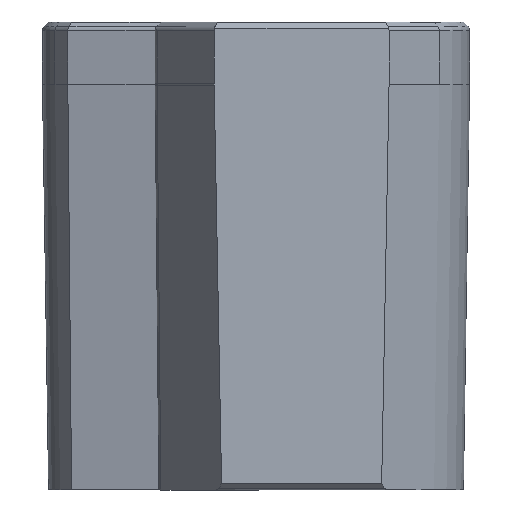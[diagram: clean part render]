
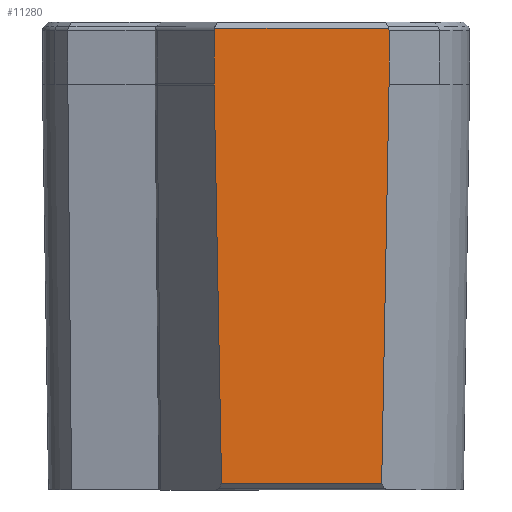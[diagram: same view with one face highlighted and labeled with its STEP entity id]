
A CAD part, left-side view. The second image highlights one B-rep face of the part: STEP entity #11280.
In plain terms, the highlighted planar face has unit normal (-1, 0, 0).
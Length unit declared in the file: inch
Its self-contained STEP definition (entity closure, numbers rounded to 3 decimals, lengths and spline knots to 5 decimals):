
#198 = CARTESIAN_POINT ( 'NONE',  ( -0.683, 0.35555, 2.003 ) ) ;
#259 = VECTOR ( 'NONE', #10219, 39.37008 ) ;
#330 = VECTOR ( 'NONE', #4020, 39.37008 ) ;
#607 = CARTESIAN_POINT ( 'NONE',  ( -0.683, -0.35555, 1.96764 ) ) ;
#680 = EDGE_CURVE ( 'NONE', #5226, #2300, #3069, .T. ) ;
#1098 = CARTESIAN_POINT ( 'NONE',  ( -0.683, -0.34029, 0.925 ) ) ;
#1530 = VERTEX_POINT ( 'NONE', #1868 ) ;
#1868 = CARTESIAN_POINT ( 'NONE',  ( -0.683, 0.35555, 1.96764 ) ) ;
#1951 = VERTEX_POINT ( 'NONE', #11167 ) ;
#2091 = DIRECTION ( 'NONE',  ( 0., 1., 0. ) ) ;
#2143 = CARTESIAN_POINT ( 'NONE',  ( -0.683, 0.35281, 1.978 ) ) ;
#2300 = VERTEX_POINT ( 'NONE', #8418 ) ;
#2865 = CARTESIAN_POINT ( 'NONE',  ( -0.683, 0.35555, 1.978 ) ) ;
#2933 = DIRECTION ( 'NONE',  ( 0., 0., -1. ) ) ;
#2955 = VERTEX_POINT ( 'NONE', #3021 ) ;
#3021 = CARTESIAN_POINT ( 'NONE',  ( -0.683, -0.35555, 1.75 ) ) ;
#3036 = AXIS2_PLACEMENT_3D ( 'NONE', #7751, #3090, #9594 ) ;
#3050 = CARTESIAN_POINT ( 'NONE',  ( -0.683, 0.32549, 0.125 ) ) ;
#3069 = LINE ( 'NONE', #5818, #330 ) ;
#3090 = DIRECTION ( 'NONE',  ( -1., 0., 0. ) ) ;
#3144 = ORIENTED_EDGE ( 'NONE', *, *, #8062, .T. ) ;
#3213 =( BOUNDED_CURVE ( )  B_SPLINE_CURVE ( 3, ( #2143, #5786, #9425, #3990 ),
 .UNSPECIFIED., .F., .T. ) 
 B_SPLINE_CURVE_WITH_KNOTS ( ( 4, 4 ),
 ( 5.85611, 6.28319 ),
 .UNSPECIFIED. ) 
 CURVE ( )  GEOMETRIC_REPRESENTATION_ITEM ( )  RATIONAL_B_SPLINE_CURVE ( ( 1., 0.985, 0.985, 1. ) ) 
 REPRESENTATION_ITEM ( '' )  );
#3379 = VERTEX_POINT ( 'NONE', #7163 ) ;
#3594 = ORIENTED_EDGE ( 'NONE', *, *, #4364, .T. ) ;
#3728 =( BOUNDED_CURVE ( )  B_SPLINE_CURVE ( 3, ( #4738, #5692, #10046, #10289 ),
 .UNSPECIFIED., .F., .T. ) 
 B_SPLINE_CURVE_WITH_KNOTS ( ( 4, 4 ),
 ( 0., 0.01515 ),
 .UNSPECIFIED. ) 
 CURVE ( )  GEOMETRIC_REPRESENTATION_ITEM ( )  RATIONAL_B_SPLINE_CURVE ( ( 1., 1., 1., 1. ) ) 
 REPRESENTATION_ITEM ( '' )  );
#3874 = ORIENTED_EDGE ( 'NONE', *, *, #5268, .F. ) ;
#3990 = CARTESIAN_POINT ( 'NONE',  ( -0.683, 0.35555, 1.96764 ) ) ;
#4020 = DIRECTION ( 'NONE',  ( 0., -1., 0. ) ) ;
#4364 = EDGE_CURVE ( 'NONE', #1951, #1530, #3213, .T. ) ;
#4727 = LINE ( 'NONE', #198, #259 ) ;
#4738 = CARTESIAN_POINT ( 'NONE',  ( -0.683, 0.35555, 1.75379 ) ) ;
#4821 = VECTOR ( 'NONE', #2933, 39.37008 ) ;
#4966 = CARTESIAN_POINT ( 'NONE',  ( -0.683, -0.35555, 1.97123 ) ) ;
#5221 = ORIENTED_EDGE ( 'NONE', *, *, #11648, .F. ) ;
#5226 = VERTEX_POINT ( 'NONE', #3050 ) ;
#5253 = EDGE_CURVE ( 'NONE', #10054, #5226, #8552, .T. ) ;
#5268 = EDGE_CURVE ( 'NONE', #8933, #2955, #8439, .T. ) ;
#5692 = CARTESIAN_POINT ( 'NONE',  ( -0.683, 0.35555, 1.75126 ) ) ;
#5786 = CARTESIAN_POINT ( 'NONE',  ( -0.683, 0.35462, 1.97474 ) ) ;
#5818 = CARTESIAN_POINT ( 'NONE',  ( -0.683, -0.32503, 0.125 ) ) ;
#6097 = CARTESIAN_POINT ( 'NONE',  ( -0.683, -0.35462, 1.97474 ) ) ;
#6282 = LINE ( 'NONE', #1098, #7989 ) ;
#6411 = CARTESIAN_POINT ( 'NONE',  ( -0.683, 0.35555, 1.75379 ) ) ;
#6544 = EDGE_CURVE ( 'NONE', #3379, #1951, #11042, .T. ) ;
#6707 = CARTESIAN_POINT ( 'NONE',  ( -0.683, -0.35555, 2.003 ) ) ;
#7111 = VECTOR ( 'NONE', #10340, 39.37008 ) ;
#7163 = CARTESIAN_POINT ( 'NONE',  ( -0.683, -0.35281, 1.978 ) ) ;
#7381 = ORIENTED_EDGE ( 'NONE', *, *, #5253, .T. ) ;
#7686 = ORIENTED_EDGE ( 'NONE', *, *, #7772, .T. ) ;
#7751 = CARTESIAN_POINT ( 'NONE',  ( -0.683, -0.35555, 1.75 ) ) ;
#7759 = VERTEX_POINT ( 'NONE', #6411 ) ;
#7772 = EDGE_CURVE ( 'NONE', #7759, #10054, #3728, .T. ) ;
#7970 = ORIENTED_EDGE ( 'NONE', *, *, #9845, .T. ) ;
#7989 = VECTOR ( 'NONE', #9917, 39.37008 ) ;
#8062 = EDGE_CURVE ( 'NONE', #8933, #3379, #11055, .T. ) ;
#8418 = CARTESIAN_POINT ( 'NONE',  ( -0.683, -0.32549, 0.125 ) ) ;
#8439 = LINE ( 'NONE', #6707, #4821 ) ;
#8530 = FACE_OUTER_BOUND ( 'NONE', #9222, .T. ) ;
#8552 = LINE ( 'NONE', #9382, #7111 ) ;
#8933 = VERTEX_POINT ( 'NONE', #10229 ) ;
#9096 = ORIENTED_EDGE ( 'NONE', *, *, #680, .T. ) ;
#9222 = EDGE_LOOP ( 'NONE', ( #7970, #7686, #7381, #9096, #5221, #3874, #3144, #9751, #3594 ) ) ;
#9382 = CARTESIAN_POINT ( 'NONE',  ( -0.683, 0.34029, 0.925 ) ) ;
#9425 = CARTESIAN_POINT ( 'NONE',  ( -0.683, 0.35555, 1.97123 ) ) ;
#9555 = VECTOR ( 'NONE', #2091, 39.37008 ) ;
#9594 = DIRECTION ( 'NONE',  ( 0., 1., 0. ) ) ;
#9751 = ORIENTED_EDGE ( 'NONE', *, *, #6544, .T. ) ;
#9845 = EDGE_CURVE ( 'NONE', #1530, #7759, #4727, .T. ) ;
#9917 = DIRECTION ( 'NONE',  ( 0., 0.018, -1. ) ) ;
#10046 = CARTESIAN_POINT ( 'NONE',  ( -0.683, 0.35552, 1.74874 ) ) ;
#10054 = VERTEX_POINT ( 'NONE', #10845 ) ;
#10219 = DIRECTION ( 'NONE',  ( 0., 0., -1. ) ) ;
#10229 = CARTESIAN_POINT ( 'NONE',  ( -0.683, -0.35555, 1.96764 ) ) ;
#10289 = CARTESIAN_POINT ( 'NONE',  ( -0.683, 0.35548, 1.74621 ) ) ;
#10340 = DIRECTION ( 'NONE',  ( 0., -0.018, -1. ) ) ;
#10405 = CARTESIAN_POINT ( 'NONE',  ( -0.683, -0.35281, 1.978 ) ) ;
#10845 = CARTESIAN_POINT ( 'NONE',  ( -0.683, 0.35548, 1.74621 ) ) ;
#11042 = LINE ( 'NONE', #2865, #9555 ) ;
#11055 =( BOUNDED_CURVE ( )  B_SPLINE_CURVE ( 3, ( #607, #4966, #6097, #10405 ),
 .UNSPECIFIED., .F., .T. ) 
 B_SPLINE_CURVE_WITH_KNOTS ( ( 4, 4 ),
 ( 3.14159, 3.56867 ),
 .UNSPECIFIED. ) 
 CURVE ( )  GEOMETRIC_REPRESENTATION_ITEM ( )  RATIONAL_B_SPLINE_CURVE ( ( 1., 0.985, 0.985, 1. ) ) 
 REPRESENTATION_ITEM ( '' )  );
#11167 = CARTESIAN_POINT ( 'NONE',  ( -0.683, 0.35281, 1.978 ) ) ;
#11205 = PLANE ( 'NONE',  #3036 ) ;
#11280 = ADVANCED_FACE ( 'NONE', ( #8530 ), #11205, .T. ) ;
#11648 = EDGE_CURVE ( 'NONE', #2955, #2300, #6282, .T. ) ;
